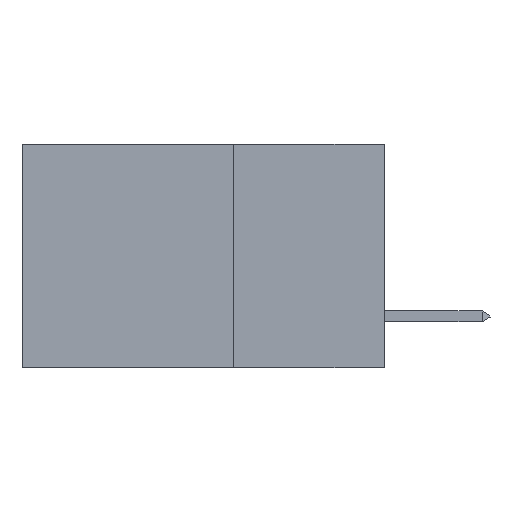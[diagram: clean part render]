
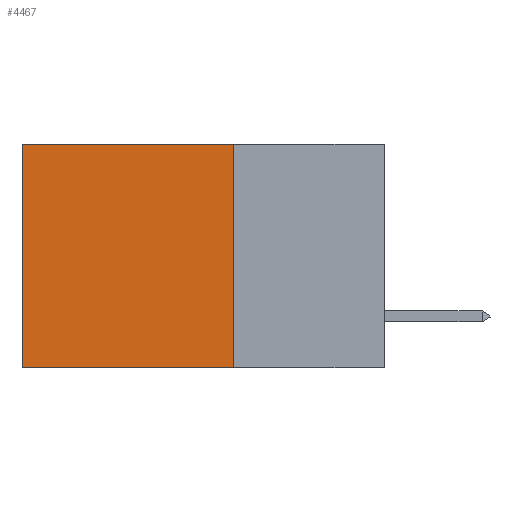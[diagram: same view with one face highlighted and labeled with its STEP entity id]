
A CAD part, left-side view. The second image highlights one B-rep face of the part: STEP entity #4467.
In plain terms, the highlighted planar face has unit normal (-1, 0, 0).
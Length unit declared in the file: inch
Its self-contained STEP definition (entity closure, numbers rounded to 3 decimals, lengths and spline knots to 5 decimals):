
#83 = CARTESIAN_POINT ( 'NONE',  ( 0.2875, 0.25, 0. ) ) ;
#1791 = CARTESIAN_POINT ( 'NONE',  ( 0.2875, 0.6, 0. ) ) ;
#3411 = CARTESIAN_POINT ( 'NONE',  ( 0.2875, 0.25, -0.37 ) ) ;
#3825 = FACE_OUTER_BOUND ( 'NONE', #18906, .T. ) ;
#4467 = ADVANCED_FACE ( 'NONE', ( #3825 ), #32512, .F. ) ;
#4535 = LINE ( 'NONE', #12307, #9692 ) ;
#6459 = VECTOR ( 'NONE', #29751, 39.37008 ) ;
#6676 = ORIENTED_EDGE ( 'NONE', *, *, #9256, .T. ) ;
#7691 = EDGE_CURVE ( 'NONE', #23891, #32502, #4535, .T. ) ;
#7718 = ORIENTED_EDGE ( 'NONE', *, *, #27639, .F. ) ;
#9256 = EDGE_CURVE ( 'NONE', #14091, #11687, #11587, .T. ) ;
#9345 = CARTESIAN_POINT ( 'NONE',  ( 0.2875, 0.6, 0. ) ) ;
#9692 = VECTOR ( 'NONE', #14834, 39.37008 ) ;
#9695 = DIRECTION ( 'NONE',  ( 0., 0., -1. ) ) ;
#11587 = LINE ( 'NONE', #29854, #6459 ) ;
#11687 = VERTEX_POINT ( 'NONE', #9345 ) ;
#12307 = CARTESIAN_POINT ( 'NONE',  ( 0.2875, 0.25, -0.37 ) ) ;
#14091 = VERTEX_POINT ( 'NONE', #23641 ) ;
#14834 = DIRECTION ( 'NONE',  ( 0., 1., 0. ) ) ;
#15498 = VECTOR ( 'NONE', #29682, 39.37008 ) ;
#18906 = EDGE_LOOP ( 'NONE', ( #30637, #32113, #7718, #6676 ) ) ;
#19936 = VECTOR ( 'NONE', #25306, 39.37008 ) ;
#21877 = AXIS2_PLACEMENT_3D ( 'NONE', #27269, #22621, #9695 ) ;
#22621 = DIRECTION ( 'NONE',  ( 1., 0., 0. ) ) ;
#23641 = CARTESIAN_POINT ( 'NONE',  ( 0.2875, 0.25, 0. ) ) ;
#23891 = VERTEX_POINT ( 'NONE', #3411 ) ;
#24697 = LINE ( 'NONE', #1791, #15498 ) ;
#25306 = DIRECTION ( 'NONE',  ( 0., 0., -1. ) ) ;
#26452 = CARTESIAN_POINT ( 'NONE',  ( 0.2875, 0.6, -0.37 ) ) ;
#26782 = LINE ( 'NONE', #83, #19936 ) ;
#27269 = CARTESIAN_POINT ( 'NONE',  ( 0.2875, 0.25, 0. ) ) ;
#27639 = EDGE_CURVE ( 'NONE', #14091, #23891, #26782, .T. ) ;
#29055 = EDGE_CURVE ( 'NONE', #11687, #32502, #24697, .T. ) ;
#29682 = DIRECTION ( 'NONE',  ( 0., 0., -1. ) ) ;
#29751 = DIRECTION ( 'NONE',  ( 0., 1., 0. ) ) ;
#29854 = CARTESIAN_POINT ( 'NONE',  ( 0.2875, 0.25, 0. ) ) ;
#30637 = ORIENTED_EDGE ( 'NONE', *, *, #29055, .T. ) ;
#32113 = ORIENTED_EDGE ( 'NONE', *, *, #7691, .F. ) ;
#32502 = VERTEX_POINT ( 'NONE', #26452 ) ;
#32512 = PLANE ( 'NONE',  #21877 ) ;
